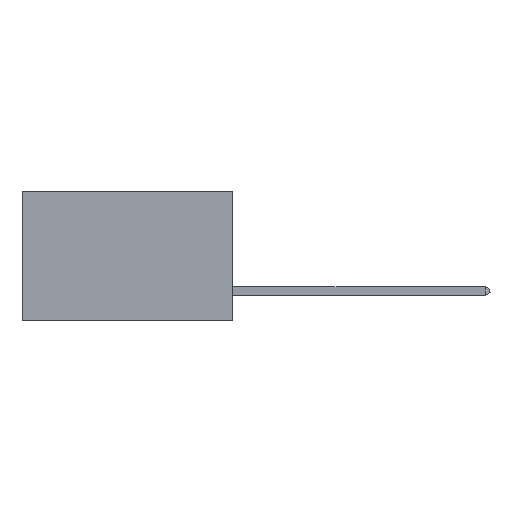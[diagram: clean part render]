
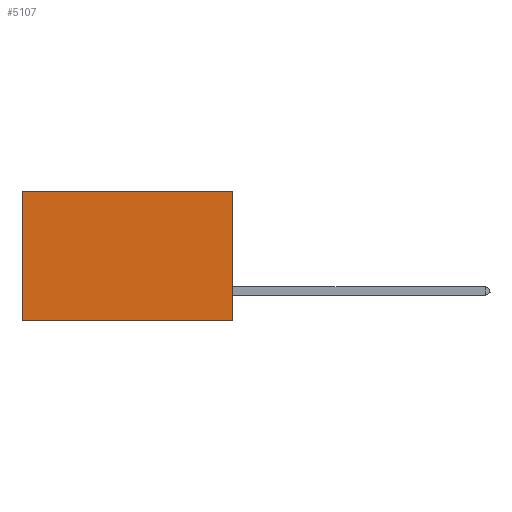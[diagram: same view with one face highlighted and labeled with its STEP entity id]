
A CAD part, left-side view. The second image highlights one B-rep face of the part: STEP entity #5107.
In plain terms, the highlighted planar face has unit normal (-1, 0, 0).
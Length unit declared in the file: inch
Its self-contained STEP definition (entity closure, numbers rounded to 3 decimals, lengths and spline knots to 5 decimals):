
#538 = VERTEX_POINT ( 'NONE', #2034 ) ;
#1043 = CARTESIAN_POINT ( 'NONE',  ( 0.2875, 0., 0. ) ) ;
#1080 = FACE_OUTER_BOUND ( 'NONE', #12021, .T. ) ;
#2034 = CARTESIAN_POINT ( 'NONE',  ( 0.2875, 0., -0.37 ) ) ;
#2229 = EDGE_CURVE ( 'NONE', #6495, #538, #13404, .T. ) ;
#3213 = CARTESIAN_POINT ( 'NONE',  ( 0.2875, 0.6, -0.37 ) ) ;
#3234 = DIRECTION ( 'NONE',  ( 0., 1., 0. ) ) ;
#4299 = EDGE_CURVE ( 'NONE', #6495, #16371, #11188, .T. ) ;
#5015 = DIRECTION ( 'NONE',  ( 0., 0., -1. ) ) ;
#5107 = ADVANCED_FACE ( 'NONE', ( #1080 ), #17727, .F. ) ;
#5716 = CARTESIAN_POINT ( 'NONE',  ( 0.2875, 0.6, 0. ) ) ;
#6139 = LINE ( 'NONE', #16964, #17716 ) ;
#6495 = VERTEX_POINT ( 'NONE', #1043 ) ;
#7365 = VECTOR ( 'NONE', #3234, 39.37008 ) ;
#7802 = VECTOR ( 'NONE', #19645, 39.37008 ) ;
#9225 = DIRECTION ( 'NONE',  ( 1., 0., 0. ) ) ;
#10305 = DIRECTION ( 'NONE',  ( 0., 1., 0. ) ) ;
#10468 = CARTESIAN_POINT ( 'NONE',  ( 0.2875, 0., 0. ) ) ;
#11188 = LINE ( 'NONE', #22147, #7365 ) ;
#11701 = CARTESIAN_POINT ( 'NONE',  ( 0.2875, 0., 0. ) ) ;
#11998 = VERTEX_POINT ( 'NONE', #3213 ) ;
#12021 = EDGE_LOOP ( 'NONE', ( #19369, #19701, #20092, #17718 ) ) ;
#12399 = LINE ( 'NONE', #5716, #7802 ) ;
#13145 = VECTOR ( 'NONE', #5015, 39.37008 ) ;
#13404 = LINE ( 'NONE', #11701, #13145 ) ;
#13717 = EDGE_CURVE ( 'NONE', #16371, #11998, #12399, .T. ) ;
#14626 = EDGE_CURVE ( 'NONE', #538, #11998, #6139, .T. ) ;
#16371 = VERTEX_POINT ( 'NONE', #21902 ) ;
#16964 = CARTESIAN_POINT ( 'NONE',  ( 0.2875, 0., -0.37 ) ) ;
#17716 = VECTOR ( 'NONE', #10305, 39.37008 ) ;
#17718 = ORIENTED_EDGE ( 'NONE', *, *, #4299, .T. ) ;
#17727 = PLANE ( 'NONE',  #18587 ) ;
#18587 = AXIS2_PLACEMENT_3D ( 'NONE', #10468, #9225, #21285 ) ;
#19369 = ORIENTED_EDGE ( 'NONE', *, *, #13717, .T. ) ;
#19645 = DIRECTION ( 'NONE',  ( 0., 0., -1. ) ) ;
#19701 = ORIENTED_EDGE ( 'NONE', *, *, #14626, .F. ) ;
#20092 = ORIENTED_EDGE ( 'NONE', *, *, #2229, .F. ) ;
#21285 = DIRECTION ( 'NONE',  ( 0., 0., -1. ) ) ;
#21902 = CARTESIAN_POINT ( 'NONE',  ( 0.2875, 0.6, 0. ) ) ;
#22147 = CARTESIAN_POINT ( 'NONE',  ( 0.2875, 0., 0. ) ) ;
